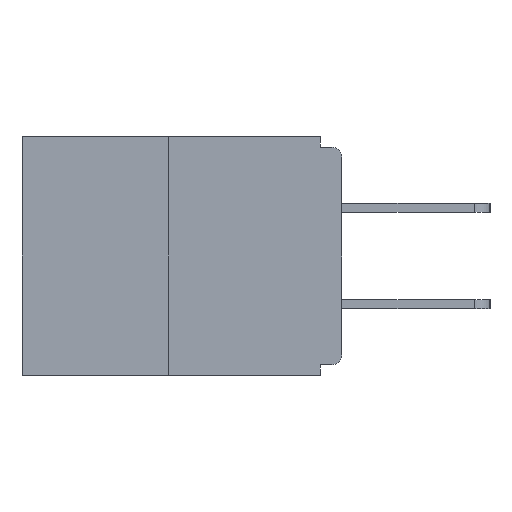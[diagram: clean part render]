
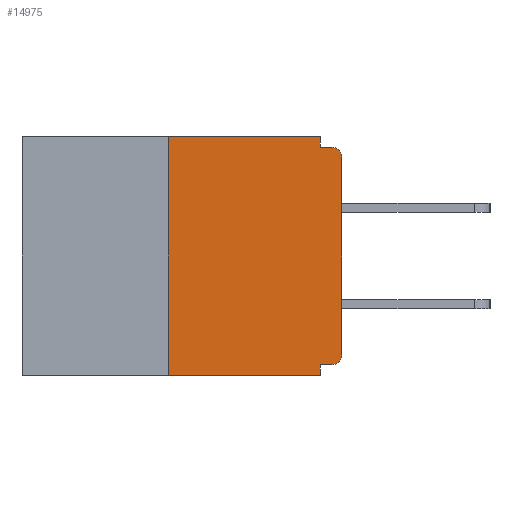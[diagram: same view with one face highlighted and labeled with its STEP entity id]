
A CAD part, left-side view. The second image highlights one B-rep face of the part: STEP entity #14975.
In plain terms, the highlighted planar face has unit normal (-1, 0, 0).
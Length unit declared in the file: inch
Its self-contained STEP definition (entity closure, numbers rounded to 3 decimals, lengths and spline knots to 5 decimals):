
#369 = EDGE_CURVE ( 'NONE', #9460, #11017, #4811, .T. ) ;
#594 = DIRECTION ( 'NONE',  ( -1., 0., 0. ) ) ;
#960 = EDGE_CURVE ( 'NONE', #11773, #9460, #16728, .T. ) ;
#1154 = AXIS2_PLACEMENT_3D ( 'NONE', #7316, #594, #12953 ) ;
#1479 = VECTOR ( 'NONE', #8883, 39.37008 ) ;
#1545 = DIRECTION ( 'NONE',  ( 0., 0., -1. ) ) ;
#2593 = VECTOR ( 'NONE', #16955, 39.37008 ) ;
#2879 = CARTESIAN_POINT ( 'NONE',  ( 0., 0.46, 0. ) ) ;
#3056 = ORIENTED_EDGE ( 'NONE', *, *, #13431, .F. ) ;
#3157 = ORIENTED_EDGE ( 'NONE', *, *, #16153, .F. ) ;
#3433 = ORIENTED_EDGE ( 'NONE', *, *, #5401, .F. ) ;
#3521 = LINE ( 'NONE', #11825, #17341 ) ;
#3629 = DIRECTION ( 'NONE',  ( 0., 1., 0. ) ) ;
#4218 = VERTEX_POINT ( 'NONE', #5709 ) ;
#4240 = CIRCLE ( 'NONE', #9947, 0.015 ) ;
#4375 = AXIS2_PLACEMENT_3D ( 'NONE', #2879, #16613, #11138 ) ;
#4382 = EDGE_CURVE ( 'NONE', #10216, #10488, #3521, .T. ) ;
#4811 = LINE ( 'NONE', #5303, #11069 ) ;
#5213 = CARTESIAN_POINT ( 'NONE',  ( 0., 0., -0.313 ) ) ;
#5303 = CARTESIAN_POINT ( 'NONE',  ( 0., 0., 0. ) ) ;
#5401 = EDGE_CURVE ( 'NONE', #11773, #4218, #7736, .T. ) ;
#5555 = CARTESIAN_POINT ( 'NONE',  ( 0., 0.25, -0.343 ) ) ;
#5625 = ORIENTED_EDGE ( 'NONE', *, *, #369, .T. ) ;
#5709 = CARTESIAN_POINT ( 'NONE',  ( 0., 0.031, -0.328 ) ) ;
#5776 = CARTESIAN_POINT ( 'NONE',  ( 0., 0.031, 0. ) ) ;
#5850 = CARTESIAN_POINT ( 'NONE',  ( 0., 0.031, -0.343 ) ) ;
#5857 = EDGE_CURVE ( 'NONE', #14671, #16590, #16654, .T. ) ;
#6253 = CARTESIAN_POINT ( 'NONE',  ( 0., 0.015, -0.015 ) ) ;
#6380 = ORIENTED_EDGE ( 'NONE', *, *, #4382, .T. ) ;
#6510 = CARTESIAN_POINT ( 'NONE',  ( 0., 0., -0.015 ) ) ;
#6599 = EDGE_CURVE ( 'NONE', #7864, #14671, #13831, .T. ) ;
#6670 = DIRECTION ( 'NONE',  ( 0., 0., 1. ) ) ;
#6846 = CARTESIAN_POINT ( 'NONE',  ( 0., 0.031, -0.343 ) ) ;
#6981 = ORIENTED_EDGE ( 'NONE', *, *, #8151, .T. ) ;
#7316 = CARTESIAN_POINT ( 'NONE',  ( 0., 0.015, -0.313 ) ) ;
#7498 = DIRECTION ( 'NONE',  ( 0., -1., 0. ) ) ;
#7736 = LINE ( 'NONE', #12130, #15127 ) ;
#7864 = VERTEX_POINT ( 'NONE', #9679 ) ;
#8151 = EDGE_CURVE ( 'NONE', #11017, #8534, #4240, .T. ) ;
#8534 = VERTEX_POINT ( 'NONE', #6253 ) ;
#8883 = DIRECTION ( 'NONE',  ( 0., 0., 1. ) ) ;
#9224 = LINE ( 'NONE', #17196, #1479 ) ;
#9442 = EDGE_LOOP ( 'NONE', ( #14191, #13252, #6380, #3157, #3433, #11388, #5625, #6981, #3056, #15784 ) ) ;
#9460 = VERTEX_POINT ( 'NONE', #5213 ) ;
#9468 = VECTOR ( 'NONE', #16537, 39.37008 ) ;
#9679 = CARTESIAN_POINT ( 'NONE',  ( 0., 0.25, 0. ) ) ;
#9812 = PLANE ( 'NONE',  #4375 ) ;
#9947 = AXIS2_PLACEMENT_3D ( 'NONE', #15914, #11986, #15850 ) ;
#9959 = CARTESIAN_POINT ( 'NONE',  ( 0., 0.46, 0. ) ) ;
#10216 = VERTEX_POINT ( 'NONE', #5555 ) ;
#10336 = LINE ( 'NONE', #5850, #11863 ) ;
#10488 = VERTEX_POINT ( 'NONE', #6846 ) ;
#10812 = CARTESIAN_POINT ( 'NONE',  ( 0., 0., -0.03 ) ) ;
#11017 = VERTEX_POINT ( 'NONE', #10812 ) ;
#11069 = VECTOR ( 'NONE', #6670, 39.37008 ) ;
#11138 = DIRECTION ( 'NONE',  ( 0., 0., -1. ) ) ;
#11388 = ORIENTED_EDGE ( 'NONE', *, *, #960, .T. ) ;
#11425 = VECTOR ( 'NONE', #14103, 39.37008 ) ;
#11773 = VERTEX_POINT ( 'NONE', #16357 ) ;
#11825 = CARTESIAN_POINT ( 'NONE',  ( 0., 0.46, -0.343 ) ) ;
#11863 = VECTOR ( 'NONE', #1545, 39.37008 ) ;
#11986 = DIRECTION ( 'NONE',  ( -1., 0., 0. ) ) ;
#12130 = CARTESIAN_POINT ( 'NONE',  ( 0., 0., -0.328 ) ) ;
#12953 = DIRECTION ( 'NONE',  ( 0., 0., -1. ) ) ;
#13252 = ORIENTED_EDGE ( 'NONE', *, *, #14544, .F. ) ;
#13431 = EDGE_CURVE ( 'NONE', #16590, #8534, #17311, .T. ) ;
#13831 = LINE ( 'NONE', #9959, #11425 ) ;
#14000 = FACE_OUTER_BOUND ( 'NONE', #9442, .T. ) ;
#14103 = DIRECTION ( 'NONE',  ( 0., -1., 0. ) ) ;
#14191 = ORIENTED_EDGE ( 'NONE', *, *, #6599, .F. ) ;
#14544 = EDGE_CURVE ( 'NONE', #10216, #7864, #9224, .T. ) ;
#14671 = VERTEX_POINT ( 'NONE', #5776 ) ;
#14975 = ADVANCED_FACE ( 'NONE', ( #14000 ), #9812, .F. ) ;
#15088 = CARTESIAN_POINT ( 'NONE',  ( 0., 0.031, 0. ) ) ;
#15127 = VECTOR ( 'NONE', #3629, 39.37008 ) ;
#15784 = ORIENTED_EDGE ( 'NONE', *, *, #5857, .F. ) ;
#15850 = DIRECTION ( 'NONE',  ( 0., 0., -1. ) ) ;
#15914 = CARTESIAN_POINT ( 'NONE',  ( 0., 0.015, -0.03 ) ) ;
#16153 = EDGE_CURVE ( 'NONE', #4218, #10488, #10336, .T. ) ;
#16357 = CARTESIAN_POINT ( 'NONE',  ( 0., 0.015, -0.328 ) ) ;
#16537 = DIRECTION ( 'NONE',  ( 0., 0., -1. ) ) ;
#16590 = VERTEX_POINT ( 'NONE', #17416 ) ;
#16613 = DIRECTION ( 'NONE',  ( 1., 0., 0. ) ) ;
#16654 = LINE ( 'NONE', #15088, #9468 ) ;
#16728 = CIRCLE ( 'NONE', #1154, 0.015 ) ;
#16955 = DIRECTION ( 'NONE',  ( 0., -1., 0. ) ) ;
#17196 = CARTESIAN_POINT ( 'NONE',  ( 0., 0.25, 0. ) ) ;
#17311 = LINE ( 'NONE', #6510, #2593 ) ;
#17341 = VECTOR ( 'NONE', #7498, 39.37008 ) ;
#17416 = CARTESIAN_POINT ( 'NONE',  ( 0., 0.031, -0.015 ) ) ;
